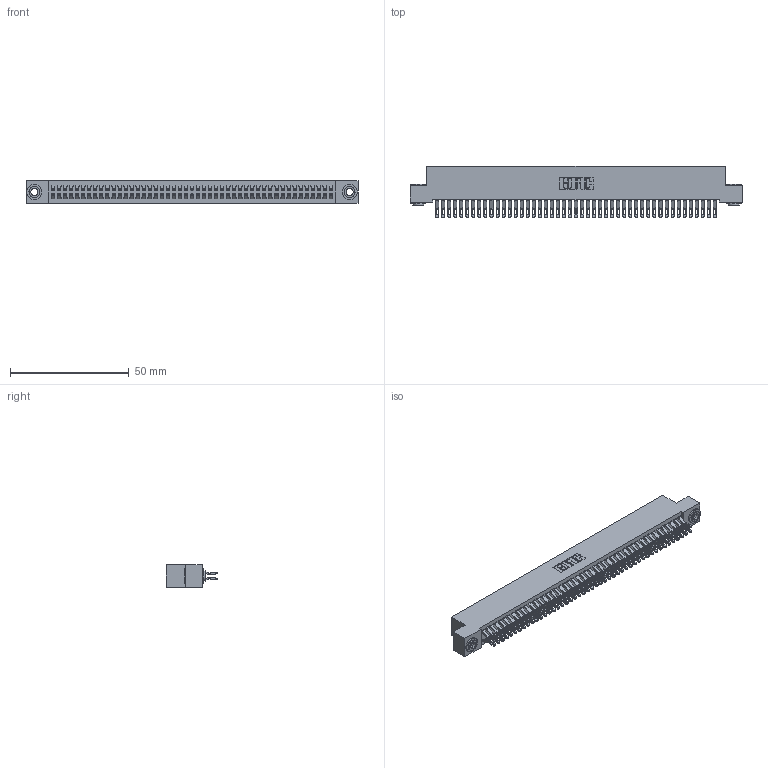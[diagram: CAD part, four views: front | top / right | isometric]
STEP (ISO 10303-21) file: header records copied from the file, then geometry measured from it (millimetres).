
FILE_DESCRIPTION (( 'STEP AP203' ), '1' );
FILE_NAME ('342-094-555-203.STEP', '2018-08-14T02:39:09', ( '' ), ( '' ), 'SwSTEP 2.0', 'SolidWorks 2016', '' );
FILE_SCHEMA (( 'CONFIG_CONTROL_DESIGN' ));
Length unit declared in the file: inch
Products named in the file (4): 345-292-001_555 Tail; 342-250-002_345-250-002-102; 342-094-555-203; 342 Part_.156 TH
Assembly tree (97 placements, depth 2):
  342-094-555-203
    342 Part_.156 TH
    345-292-001_555 Tail  x94
    342-250-002_345-250-002-102  x2
Bounding box: 139.7 x 21.47 x 9.4 mm (x, y, z)
Volume: 12859.7 mm3; surface area: 22179.2 mm2
Topology: 97 solids, 97 shells, 5600 faces, 17577 edges, 11714 vertices
Faces by surface type: plane 3272, cylinder 2320, cone 8
Entity records: 30434 total; most frequent: CARTESIAN_POINT 5047, ORIENTED_EDGE 4946, DIRECTION 4307, EDGE_CURVE 2473, VECTOR 2301, LINE 2301, VERTEX_POINT 1646, AXIS2_PLACEMENT_3D 1003
